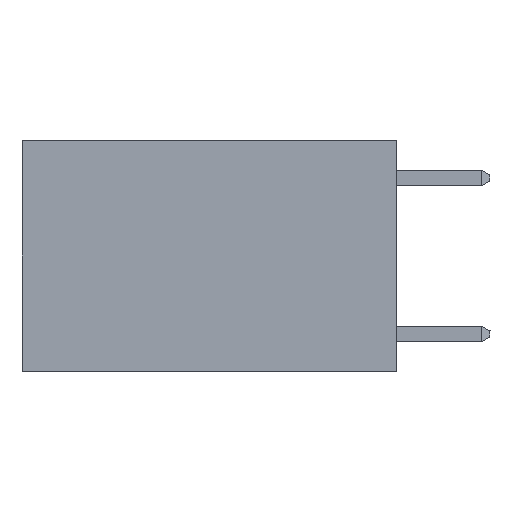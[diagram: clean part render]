
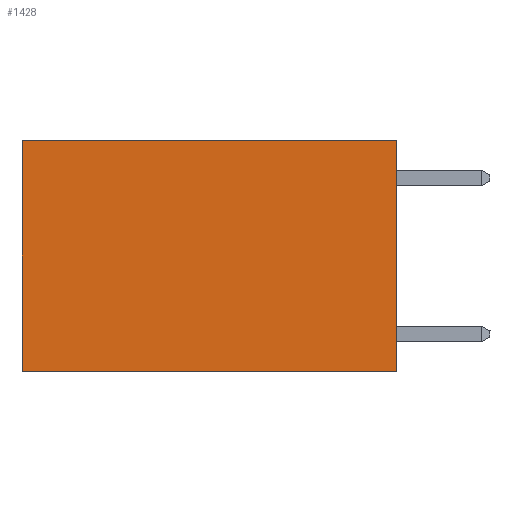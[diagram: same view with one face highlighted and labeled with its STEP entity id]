
A CAD part, left-side view. The second image highlights one B-rep face of the part: STEP entity #1428.
In plain terms, the highlighted planar face has unit normal (-1, 0, 0).
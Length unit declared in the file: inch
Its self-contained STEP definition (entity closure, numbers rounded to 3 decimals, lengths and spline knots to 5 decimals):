
#214 = VECTOR ( 'NONE', #10267, 39.37008 ) ;
#226 = AXIS2_PLACEMENT_3D ( 'NONE', #3637, #10103, #6821 ) ;
#939 = LINE ( 'NONE', #9474, #10738 ) ;
#963 = LINE ( 'NONE', #1086, #10403 ) ;
#1086 = CARTESIAN_POINT ( 'NONE',  ( 0.2625, 0., -0.37 ) ) ;
#1428 = ADVANCED_FACE ( 'NONE', ( #8131 ), #8445, .F. ) ;
#1515 = VERTEX_POINT ( 'NONE', #10665 ) ;
#2139 = DIRECTION ( 'NONE',  ( 0., 0., -1. ) ) ;
#2382 = CARTESIAN_POINT ( 'NONE',  ( 0.2625, 0., 0. ) ) ;
#2869 = VECTOR ( 'NONE', #4819, 39.37008 ) ;
#3637 = CARTESIAN_POINT ( 'NONE',  ( 0.2625, 0., 0. ) ) ;
#4819 = DIRECTION ( 'NONE',  ( 0., 1., 0. ) ) ;
#4885 = VERTEX_POINT ( 'NONE', #15564 ) ;
#4925 = EDGE_CURVE ( 'NONE', #1515, #6178, #9382, .T. ) ;
#5446 = CARTESIAN_POINT ( 'NONE',  ( 0.2625, 0.6, -0.37 ) ) ;
#5605 = ORIENTED_EDGE ( 'NONE', *, *, #8117, .F. ) ;
#5981 = ORIENTED_EDGE ( 'NONE', *, *, #4925, .T. ) ;
#6178 = VERTEX_POINT ( 'NONE', #10671 ) ;
#6372 = LINE ( 'NONE', #9029, #214 ) ;
#6821 = DIRECTION ( 'NONE',  ( 0., 0., -1. ) ) ;
#8117 = EDGE_CURVE ( 'NONE', #1515, #4885, #6372, .T. ) ;
#8131 = FACE_OUTER_BOUND ( 'NONE', #15349, .T. ) ;
#8445 = PLANE ( 'NONE',  #226 ) ;
#8456 = DIRECTION ( 'NONE',  ( 0., 1., 0. ) ) ;
#9029 = CARTESIAN_POINT ( 'NONE',  ( 0.2625, 0., 0. ) ) ;
#9382 = LINE ( 'NONE', #2382, #2869 ) ;
#9473 = VERTEX_POINT ( 'NONE', #5446 ) ;
#9474 = CARTESIAN_POINT ( 'NONE',  ( 0.2625, 0.6, 0. ) ) ;
#10103 = DIRECTION ( 'NONE',  ( 1., 0., 0. ) ) ;
#10267 = DIRECTION ( 'NONE',  ( 0., 0., -1. ) ) ;
#10403 = VECTOR ( 'NONE', #8456, 39.37008 ) ;
#10665 = CARTESIAN_POINT ( 'NONE',  ( 0.2625, 0., 0. ) ) ;
#10671 = CARTESIAN_POINT ( 'NONE',  ( 0.2625, 0.6, 0. ) ) ;
#10738 = VECTOR ( 'NONE', #2139, 39.37008 ) ;
#13750 = EDGE_CURVE ( 'NONE', #4885, #9473, #963, .T. ) ;
#14510 = ORIENTED_EDGE ( 'NONE', *, *, #15119, .T. ) ;
#14913 = ORIENTED_EDGE ( 'NONE', *, *, #13750, .F. ) ;
#15119 = EDGE_CURVE ( 'NONE', #6178, #9473, #939, .T. ) ;
#15349 = EDGE_LOOP ( 'NONE', ( #14510, #14913, #5605, #5981 ) ) ;
#15564 = CARTESIAN_POINT ( 'NONE',  ( 0.2625, 0., -0.37 ) ) ;
